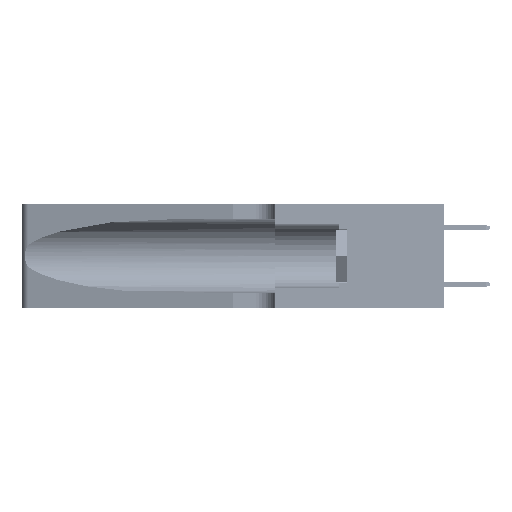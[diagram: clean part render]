
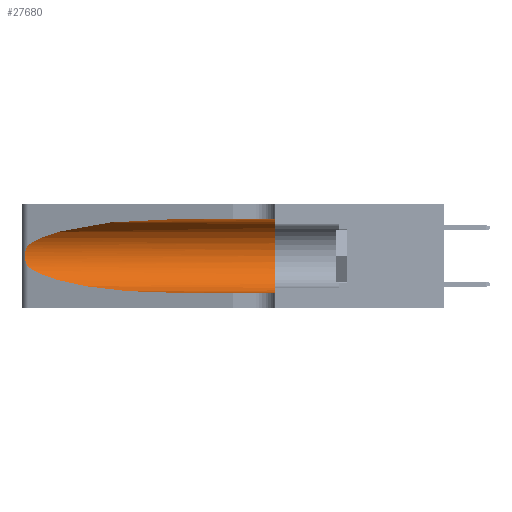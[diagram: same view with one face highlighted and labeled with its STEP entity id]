
A CAD part, left-side view. The second image highlights one B-rep face of the part: STEP entity #27680.
In plain terms, the highlighted cylindrical face has radius 3.308 mm (diameter 6.617 mm), a partial arc.
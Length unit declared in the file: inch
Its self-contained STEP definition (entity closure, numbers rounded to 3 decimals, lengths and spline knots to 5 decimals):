
#318 = ORIENTED_EDGE ( 'NONE', *, *, #28315, .F. ) ;
#1249 = VECTOR ( 'NONE', #8024, 39.37008 ) ;
#1643 = DIRECTION ( 'NONE',  ( 0., -1., 0. ) ) ;
#3263 = CARTESIAN_POINT ( 'NONE',  ( 0.25487, 1.22718, 0.22369 ) ) ;
#3469 = CARTESIAN_POINT ( 'NONE',  ( 0.25787, 1.23484, 0.2124 ) ) ;
#4142 = EDGE_CURVE ( 'NONE', #21447, #45907, #7444, .T. ) ;
#4644 = EDGE_CURVE ( 'NONE', #7159, #45907, #22187, .T. ) ;
#5289 = VECTOR ( 'NONE', #1643, 39.37008 ) ;
#5423 = CARTESIAN_POINT ( 'NONE',  ( 0.1305, 0.35, 0.05475 ) ) ;
#5642 =( BOUNDED_CURVE ( )  B_SPLINE_CURVE ( 3, ( #17653, #5768, #49033, #25564 ),
 .UNSPECIFIED., .F., .F. ) 
 B_SPLINE_CURVE_WITH_KNOTS ( ( 4, 4 ),
 ( 1.5708, 2.84003 ),
 .UNSPECIFIED. ) 
 CURVE ( )  GEOMETRIC_REPRESENTATION_ITEM ( )  RATIONAL_B_SPLINE_CURVE ( ( 1., 0.87, 0.87, 1. ) ) 
 REPRESENTATION_ITEM ( '' )  );
#5768 = CARTESIAN_POINT ( 'NONE',  ( 0.18966, 0.96281, 0.31525 ) ) ;
#7159 = VERTEX_POINT ( 'NONE', #8391 ) ;
#7410 = CARTESIAN_POINT ( 'NONE',  ( 0.26018, 1.23835, 0.19895 ) ) ;
#7444 = CIRCLE ( 'NONE', #47759, 0.13025 ) ;
#8024 = DIRECTION ( 'NONE',  ( 0., -1., 0. ) ) ;
#8337 = CARTESIAN_POINT ( 'NONE',  ( 0.1305, 0.72297, 0.31525 ) ) ;
#8391 = CARTESIAN_POINT ( 'NONE',  ( 0.1305, 0.72297, 0.05475 ) ) ;
#8764 = EDGE_CURVE ( 'NONE', #29883, #29477, #9453, .T. ) ;
#9453 = B_SPLINE_CURVE_WITH_KNOTS ( 'NONE', 3,
 ( #50509, #46564, #42618, #3469, #30973, #7410, #34879, #11382, #38849, #15348, #42786, #19308, #46727, #23262 ),
 .UNSPECIFIED., .F., .F.,
 ( 4, 2, 2, 2, 2, 2, 4 ),
 ( 0., 0.00027, 0.00053, 0.00107, 0.0016, 0.00187, 0.00214 ),
 .UNSPECIFIED. ) ;
#9773 = CARTESIAN_POINT ( 'NONE',  ( 0.1305, 1.61858, 0.185 ) ) ;
#11382 = CARTESIAN_POINT ( 'NONE',  ( 0.26075, 1.23896, 0.178 ) ) ;
#12009 = CARTESIAN_POINT ( 'NONE',  ( 0.1305, 1.61858, 0.05475 ) ) ;
#12495 = EDGE_CURVE ( 'NONE', #29477, #7159, #42176, .T. ) ;
#12917 = DIRECTION ( 'NONE',  ( 0., 1., 0. ) ) ;
#13538 = CARTESIAN_POINT ( 'NONE',  ( 0.1305, 0.72297, 0.05475 ) ) ;
#13974 = ORIENTED_EDGE ( 'NONE', *, *, #12495, .T. ) ;
#15189 = AXIS2_PLACEMENT_3D ( 'NONE', #9773, #45134, #41169 ) ;
#15348 = CARTESIAN_POINT ( 'NONE',  ( 0.25856, 1.23593, 0.16098 ) ) ;
#17653 = CARTESIAN_POINT ( 'NONE',  ( 0.1305, 0.72297, 0.31525 ) ) ;
#17701 = FACE_OUTER_BOUND ( 'NONE', #48770, .T. ) ;
#19308 = CARTESIAN_POINT ( 'NONE',  ( 0.25639, 1.23186, 0.15144 ) ) ;
#19348 = ORIENTED_EDGE ( 'NONE', *, *, #4142, .F. ) ;
#21447 = VERTEX_POINT ( 'NONE', #49881 ) ;
#22187 = LINE ( 'NONE', #12009, #1249 ) ;
#22675 = ORIENTED_EDGE ( 'NONE', *, *, #33836, .T. ) ;
#23262 = CARTESIAN_POINT ( 'NONE',  ( 0.25487, 1.22718, 0.14631 ) ) ;
#25564 = CARTESIAN_POINT ( 'NONE',  ( 0.25487, 1.22718, 0.22369 ) ) ;
#27453 = LINE ( 'NONE', #48677, #5289 ) ;
#27680 = ADVANCED_FACE ( 'NONE', ( #17701 ), #45316, .F. ) ;
#28315 = EDGE_CURVE ( 'NONE', #48149, #21447, #27453, .T. ) ;
#29477 = VERTEX_POINT ( 'NONE', #44155 ) ;
#29847 = ORIENTED_EDGE ( 'NONE', *, *, #4644, .T. ) ;
#29883 = VERTEX_POINT ( 'NONE', #3263 ) ;
#30973 = CARTESIAN_POINT ( 'NONE',  ( 0.25854, 1.2359, 0.20912 ) ) ;
#33102 = CARTESIAN_POINT ( 'NONE',  ( 0.25487, 1.22718, 0.14631 ) ) ;
#33836 = EDGE_CURVE ( 'NONE', #48149, #29883, #5642, .T. ) ;
#34879 = CARTESIAN_POINT ( 'NONE',  ( 0.26075, 1.23896, 0.19203 ) ) ;
#36401 = CARTESIAN_POINT ( 'NONE',  ( 0.1305, 0.35, 0.185 ) ) ;
#37038 = CARTESIAN_POINT ( 'NONE',  ( 0.18966, 0.96281, 0.05475 ) ) ;
#38823 = ORIENTED_EDGE ( 'NONE', *, *, #8764, .T. ) ;
#38849 = CARTESIAN_POINT ( 'NONE',  ( 0.26017, 1.23833, 0.17102 ) ) ;
#40361 = DIRECTION ( 'NONE',  ( 0., 0., 1. ) ) ;
#41169 = DIRECTION ( 'NONE',  ( 0., 0., -1. ) ) ;
#42176 =( BOUNDED_CURVE ( )  B_SPLINE_CURVE ( 3, ( #33102, #48724, #37038, #13538 ),
 .UNSPECIFIED., .F., .T. ) 
 B_SPLINE_CURVE_WITH_KNOTS ( ( 4, 4 ),
 ( 3.44316, 4.71239 ),
 .UNSPECIFIED. ) 
 CURVE ( )  GEOMETRIC_REPRESENTATION_ITEM ( )  RATIONAL_B_SPLINE_CURVE ( ( 1., 0.87, 0.87, 1. ) ) 
 REPRESENTATION_ITEM ( '' )  );
#42618 = CARTESIAN_POINT ( 'NONE',  ( 0.25639, 1.23184, 0.21858 ) ) ;
#42786 = CARTESIAN_POINT ( 'NONE',  ( 0.25789, 1.23486, 0.15765 ) ) ;
#44155 = CARTESIAN_POINT ( 'NONE',  ( 0.25487, 1.22718, 0.14631 ) ) ;
#45134 = DIRECTION ( 'NONE',  ( 0., -1., 0. ) ) ;
#45316 = CYLINDRICAL_SURFACE ( 'NONE', #15189, 0.13025 ) ;
#45907 = VERTEX_POINT ( 'NONE', #5423 ) ;
#46564 = CARTESIAN_POINT ( 'NONE',  ( 0.25555, 1.22994, 0.2215 ) ) ;
#46727 = CARTESIAN_POINT ( 'NONE',  ( 0.25555, 1.22993, 0.14849 ) ) ;
#47759 = AXIS2_PLACEMENT_3D ( 'NONE', #36401, #12917, #40361 ) ;
#48149 = VERTEX_POINT ( 'NONE', #8337 ) ;
#48677 = CARTESIAN_POINT ( 'NONE',  ( 0.1305, 1.61858, 0.31525 ) ) ;
#48724 = CARTESIAN_POINT ( 'NONE',  ( 0.2373, 1.15595, 0.08982 ) ) ;
#48770 = EDGE_LOOP ( 'NONE', ( #22675, #38823, #13974, #29847, #19348, #318 ) ) ;
#49033 = CARTESIAN_POINT ( 'NONE',  ( 0.2373, 1.15595, 0.28018 ) ) ;
#49881 = CARTESIAN_POINT ( 'NONE',  ( 0.1305, 0.35, 0.31525 ) ) ;
#50509 = CARTESIAN_POINT ( 'NONE',  ( 0.25487, 1.22718, 0.22369 ) ) ;
